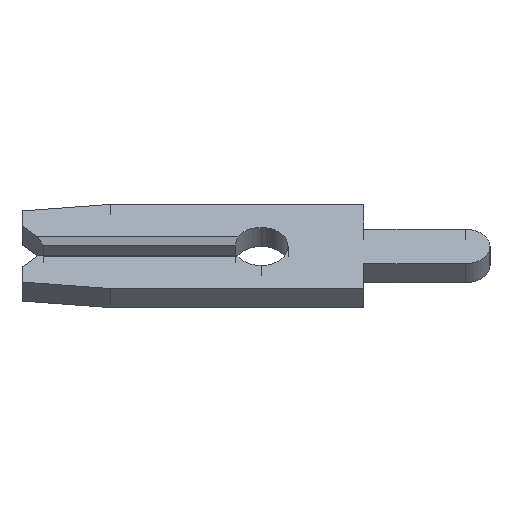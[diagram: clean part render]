
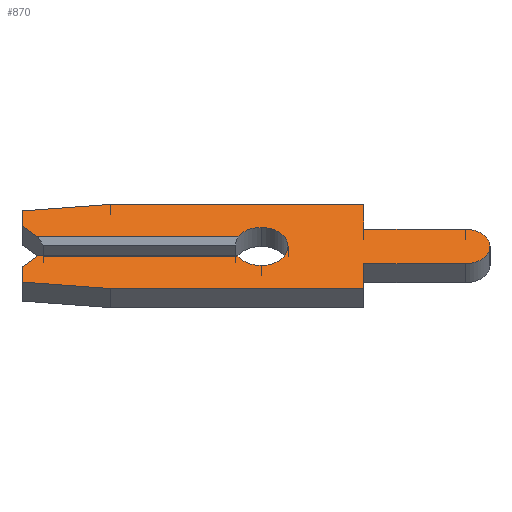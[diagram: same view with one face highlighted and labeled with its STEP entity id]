
A CAD part, left-side view. The second image highlights one B-rep face of the part: STEP entity #870.
In plain terms, the highlighted face is planar.
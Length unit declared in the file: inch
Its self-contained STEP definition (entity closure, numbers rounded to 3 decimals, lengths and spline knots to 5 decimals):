
#3 = CARTESIAN_POINT ( 'NONE',  ( -0.013, -0.099, 0.0235 ) ) ;
#17 = VERTEX_POINT ( 'NONE', #1803 ) ;
#29 = AXIS2_PLACEMENT_3D ( 'NONE', #374, #968, #1231 ) ;
#36 = VECTOR ( 'NONE', #57, 39.37008 ) ;
#37 = CARTESIAN_POINT ( 'NONE',  ( -0.013, 0.2105, -0.0075 ) ) ;
#46 = CARTESIAN_POINT ( 'NONE',  ( -0.013, -0.099, -0.0235 ) ) ;
#57 = DIRECTION ( 'NONE',  ( 0., 0.707, 0.707 ) ) ;
#64 = VECTOR ( 'NONE', #1075, 39.37008 ) ;
#78 = CARTESIAN_POINT ( 'NONE',  ( -0.013, 0.231, 0.028 ) ) ;
#82 = EDGE_CURVE ( 'NONE', #269, #252, #1210, .T. ) ;
#83 = CARTESIAN_POINT ( 'NONE',  ( -0.013, 0.146, -0.0575 ) ) ;
#84 = LINE ( 'NONE', #205, #494 ) ;
#89 = VERTEX_POINT ( 'NONE', #668 ) ;
#122 = ORIENTED_EDGE ( 'NONE', *, *, #1216, .F. ) ;
#126 = VERTEX_POINT ( 'NONE', #1423 ) ;
#157 = CARTESIAN_POINT ( 'NONE',  ( -0.013, 0., -0.026 ) ) ;
#168 = CARTESIAN_POINT ( 'NONE',  ( -0.013, -0.099, 0.0235 ) ) ;
#190 = CARTESIAN_POINT ( 'NONE',  ( -0.013, 0.146, 0.0575 ) ) ;
#205 = CARTESIAN_POINT ( 'NONE',  ( -0.013, 0., -0.013 ) ) ;
#209 = ORIENTED_EDGE ( 'NONE', *, *, #577, .F. ) ;
#210 = VERTEX_POINT ( 'NONE', #3 ) ;
#225 = VERTEX_POINT ( 'NONE', #837 ) ;
#246 = VECTOR ( 'NONE', #881, 39.37008 ) ;
#252 = VERTEX_POINT ( 'NONE', #1272 ) ;
#264 = CARTESIAN_POINT ( 'NONE',  ( -0.013, 0.02252, -0.013 ) ) ;
#269 = VERTEX_POINT ( 'NONE', #157 ) ;
#271 = VERTEX_POINT ( 'NONE', #1567 ) ;
#290 = LINE ( 'NONE', #37, #595 ) ;
#293 = ORIENTED_EDGE ( 'NONE', *, *, #1570, .F. ) ;
#294 = CARTESIAN_POINT ( 'NONE',  ( -0.013, 0.02252, 0.013 ) ) ;
#296 = ORIENTED_EDGE ( 'NONE', *, *, #657, .F. ) ;
#309 = CARTESIAN_POINT ( 'NONE',  ( -0.013, -0.1975, -0.0235 ) ) ;
#324 = CIRCLE ( 'NONE', #1512, 0.0235 ) ;
#340 = VECTOR ( 'NONE', #612, 39.37008 ) ;
#342 = LINE ( 'NONE', #923, #1425 ) ;
#349 = AXIS2_PLACEMENT_3D ( 'NONE', #460, #1599, #730 ) ;
#352 = CARTESIAN_POINT ( 'NONE',  ( -0.013, -0.099, -0.0575 ) ) ;
#355 = DIRECTION ( 'NONE',  ( 0., 0.995, 0.105 ) ) ;
#359 = CARTESIAN_POINT ( 'NONE',  ( -0.013, -0.1975, 0. ) ) ;
#365 = ORIENTED_EDGE ( 'NONE', *, *, #1130, .F. ) ;
#374 = CARTESIAN_POINT ( 'NONE',  ( -0.013, 0., 0. ) ) ;
#388 = ORIENTED_EDGE ( 'NONE', *, *, #646, .F. ) ;
#400 = DIRECTION ( 'NONE',  ( -1., 0., 0. ) ) ;
#407 = LINE ( 'NONE', #352, #1377 ) ;
#411 = LINE ( 'NONE', #1085, #616 ) ;
#460 = CARTESIAN_POINT ( 'NONE',  ( -0.013, 0., 0. ) ) ;
#474 = VERTEX_POINT ( 'NONE', #264 ) ;
#476 = ORIENTED_EDGE ( 'NONE', *, *, #1026, .T. ) ;
#477 = CARTESIAN_POINT ( 'NONE',  ( -0.013, 0.216, -0.013 ) ) ;
#490 = DIRECTION ( 'NONE',  ( 0., -1., 0. ) ) ;
#494 = VECTOR ( 'NONE', #490, 39.37008 ) ;
#498 = ORIENTED_EDGE ( 'NONE', *, *, #1367, .F. ) ;
#499 = DIRECTION ( 'NONE',  ( 0., -0.995, 0.105 ) ) ;
#522 = VERTEX_POINT ( 'NONE', #294 ) ;
#546 = VERTEX_POINT ( 'NONE', #309 ) ;
#549 = VERTEX_POINT ( 'NONE', #1717 ) ;
#571 = EDGE_LOOP ( 'NONE', ( #476, #296, #1015, #639, #1124, #122, #1303, #1236, #365, #1190, #1720, #293, #209, #388, #1195, #1696, #877, #498 ) ) ;
#577 = EDGE_CURVE ( 'NONE', #210, #681, #656, .T. ) ;
#587 = DIRECTION ( 'NONE',  ( 0., 0., -1. ) ) ;
#595 = VECTOR ( 'NONE', #1029, 39.37008 ) ;
#603 = CARTESIAN_POINT ( 'NONE',  ( -0.013, -0.099, 0.0575 ) ) ;
#612 = DIRECTION ( 'NONE',  ( 0., 1., 0. ) ) ;
#613 = EDGE_CURVE ( 'NONE', #546, #89, #1761, .T. ) ;
#616 = VECTOR ( 'NONE', #931, 39.37008 ) ;
#619 = VERTEX_POINT ( 'NONE', #1168 ) ;
#635 = VECTOR ( 'NONE', #587, 39.37008 ) ;
#636 = CARTESIAN_POINT ( 'NONE',  ( -0.013, -0.099, -0.0575 ) ) ;
#638 = AXIS2_PLACEMENT_3D ( 'NONE', #1373, #400, #1011 ) ;
#639 = ORIENTED_EDGE ( 'NONE', *, *, #1608, .F. ) ;
#646 = EDGE_CURVE ( 'NONE', #17, #210, #1609, .T. ) ;
#656 = LINE ( 'NONE', #168, #246 ) ;
#657 = EDGE_CURVE ( 'NONE', #252, #522, #1374, .T. ) ;
#668 = CARTESIAN_POINT ( 'NONE',  ( -0.013, -0.099, -0.0235 ) ) ;
#681 = VERTEX_POINT ( 'NONE', #1584 ) ;
#686 = LINE ( 'NONE', #78, #1409 ) ;
#730 = DIRECTION ( 'NONE',  ( 0., 0., -1. ) ) ;
#757 = CARTESIAN_POINT ( 'NONE',  ( -0.013, 0.2105, 0.0075 ) ) ;
#785 = VERTEX_POINT ( 'NONE', #909 ) ;
#793 = EDGE_CURVE ( 'NONE', #949, #474, #84, .T. ) ;
#837 = CARTESIAN_POINT ( 'NONE',  ( -0.013, 0.146, -0.0575 ) ) ;
#870 = ADVANCED_FACE ( 'NONE', ( #1739 ), #1773, .F. ) ;
#877 = ORIENTED_EDGE ( 'NONE', *, *, #1560, .F. ) ;
#881 = DIRECTION ( 'NONE',  ( 0., -1., 0. ) ) ;
#909 = CARTESIAN_POINT ( 'NONE',  ( -0.013, 0.216, 0.013 ) ) ;
#918 = CARTESIAN_POINT ( 'NONE',  ( -0.013, 0.231, -0.028 ) ) ;
#923 = CARTESIAN_POINT ( 'NONE',  ( -0.013, 0.231, 0.04857 ) ) ;
#924 = LINE ( 'NONE', #757, #36 ) ;
#931 = DIRECTION ( 'NONE',  ( 0., -1., 0. ) ) ;
#933 = DIRECTION ( 'NONE',  ( 0., 0., -1. ) ) ;
#949 = VERTEX_POINT ( 'NONE', #477 ) ;
#968 = DIRECTION ( 'NONE',  ( -1., 0., 0. ) ) ;
#1011 = DIRECTION ( 'NONE',  ( 0., 0., -1. ) ) ;
#1015 = ORIENTED_EDGE ( 'NONE', *, *, #82, .F. ) ;
#1026 = EDGE_CURVE ( 'NONE', #785, #522, #411, .T. ) ;
#1029 = DIRECTION ( 'NONE',  ( 0., -0.707, 0.707 ) ) ;
#1045 = CARTESIAN_POINT ( 'NONE',  ( -0.013, 0.231, -0.028 ) ) ;
#1063 = EDGE_CURVE ( 'NONE', #225, #549, #1366, .T. ) ;
#1075 = DIRECTION ( 'NONE',  ( 0., 1., 0. ) ) ;
#1080 = LINE ( 'NONE', #83, #64 ) ;
#1085 = CARTESIAN_POINT ( 'NONE',  ( -0.013, 0.231, 0.013 ) ) ;
#1086 = CIRCLE ( 'NONE', #29, 0.026 ) ;
#1124 = ORIENTED_EDGE ( 'NONE', *, *, #793, .F. ) ;
#1130 = EDGE_CURVE ( 'NONE', #1633, #225, #1080, .T. ) ;
#1168 = CARTESIAN_POINT ( 'NONE',  ( -0.013, 0.146, 0.0575 ) ) ;
#1190 = ORIENTED_EDGE ( 'NONE', *, *, #1436, .F. ) ;
#1195 = ORIENTED_EDGE ( 'NONE', *, *, #1308, .F. ) ;
#1198 = DIRECTION ( 'NONE',  ( 0., 0., 1. ) ) ;
#1207 = DIRECTION ( 'NONE',  ( 0., 0., 1. ) ) ;
#1209 = LINE ( 'NONE', #1045, #1359 ) ;
#1210 = CIRCLE ( 'NONE', #638, 0.026 ) ;
#1216 = EDGE_CURVE ( 'NONE', #1569, #949, #290, .T. ) ;
#1231 = DIRECTION ( 'NONE',  ( 0., 0., -1. ) ) ;
#1236 = ORIENTED_EDGE ( 'NONE', *, *, #1063, .F. ) ;
#1250 = VECTOR ( 'NONE', #1324, 39.37008 ) ;
#1272 = CARTESIAN_POINT ( 'NONE',  ( -0.013, 0., 0.026 ) ) ;
#1303 = ORIENTED_EDGE ( 'NONE', *, *, #1398, .F. ) ;
#1308 = EDGE_CURVE ( 'NONE', #619, #17, #1318, .T. ) ;
#1318 = LINE ( 'NONE', #190, #1250 ) ;
#1323 = DIRECTION ( 'NONE',  ( 1., 0., 0. ) ) ;
#1324 = DIRECTION ( 'NONE',  ( 0., -1., 0. ) ) ;
#1332 = AXIS2_PLACEMENT_3D ( 'NONE', #1611, #1323, #1767 ) ;
#1359 = VECTOR ( 'NONE', #1616, 39.37008 ) ;
#1366 = LINE ( 'NONE', #1637, #1434 ) ;
#1367 = EDGE_CURVE ( 'NONE', #785, #126, #924, .T. ) ;
#1373 = CARTESIAN_POINT ( 'NONE',  ( -0.013, 0., 0. ) ) ;
#1374 = CIRCLE ( 'NONE', #349, 0.026 ) ;
#1377 = VECTOR ( 'NONE', #933, 39.37008 ) ;
#1398 = EDGE_CURVE ( 'NONE', #549, #1569, #1209, .T. ) ;
#1409 = VECTOR ( 'NONE', #1207, 39.37008 ) ;
#1423 = CARTESIAN_POINT ( 'NONE',  ( -0.013, 0.231, 0.028 ) ) ;
#1425 = VECTOR ( 'NONE', #499, 39.37008 ) ;
#1434 = VECTOR ( 'NONE', #355, 39.37008 ) ;
#1436 = EDGE_CURVE ( 'NONE', #89, #1633, #407, .T. ) ;
#1449 = EDGE_CURVE ( 'NONE', #271, #619, #342, .T. ) ;
#1490 = DIRECTION ( 'NONE',  ( 1., 0., 0. ) ) ;
#1512 = AXIS2_PLACEMENT_3D ( 'NONE', #359, #1490, #1198 ) ;
#1560 = EDGE_CURVE ( 'NONE', #126, #271, #686, .T. ) ;
#1567 = CARTESIAN_POINT ( 'NONE',  ( -0.013, 0.231, 0.04857 ) ) ;
#1569 = VERTEX_POINT ( 'NONE', #918 ) ;
#1570 = EDGE_CURVE ( 'NONE', #681, #546, #324, .T. ) ;
#1584 = CARTESIAN_POINT ( 'NONE',  ( -0.013, -0.1975, 0.0235 ) ) ;
#1599 = DIRECTION ( 'NONE',  ( -1., 0., 0. ) ) ;
#1608 = EDGE_CURVE ( 'NONE', #474, #269, #1086, .T. ) ;
#1609 = LINE ( 'NONE', #603, #635 ) ;
#1611 = CARTESIAN_POINT ( 'NONE',  ( -0.013, 0., 0. ) ) ;
#1616 = DIRECTION ( 'NONE',  ( 0., 0., 1. ) ) ;
#1633 = VERTEX_POINT ( 'NONE', #636 ) ;
#1637 = CARTESIAN_POINT ( 'NONE',  ( -0.013, 0.231, -0.04857 ) ) ;
#1696 = ORIENTED_EDGE ( 'NONE', *, *, #1449, .F. ) ;
#1717 = CARTESIAN_POINT ( 'NONE',  ( -0.013, 0.231, -0.04857 ) ) ;
#1720 = ORIENTED_EDGE ( 'NONE', *, *, #613, .F. ) ;
#1739 = FACE_OUTER_BOUND ( 'NONE', #571, .T. ) ;
#1761 = LINE ( 'NONE', #46, #340 ) ;
#1767 = DIRECTION ( 'NONE',  ( 0., 0., -1. ) ) ;
#1773 = PLANE ( 'NONE',  #1332 ) ;
#1803 = CARTESIAN_POINT ( 'NONE',  ( -0.013, -0.099, 0.0575 ) ) ;
